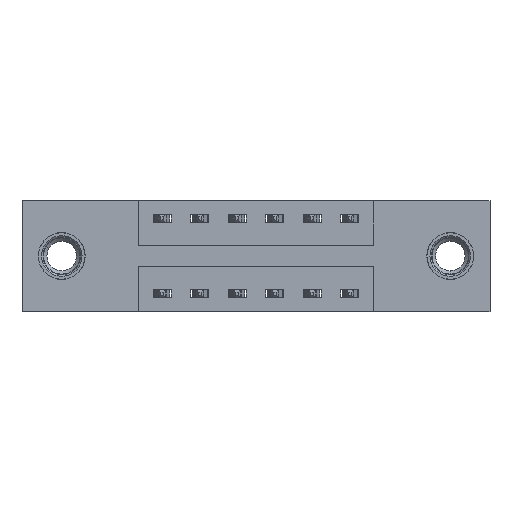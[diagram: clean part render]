
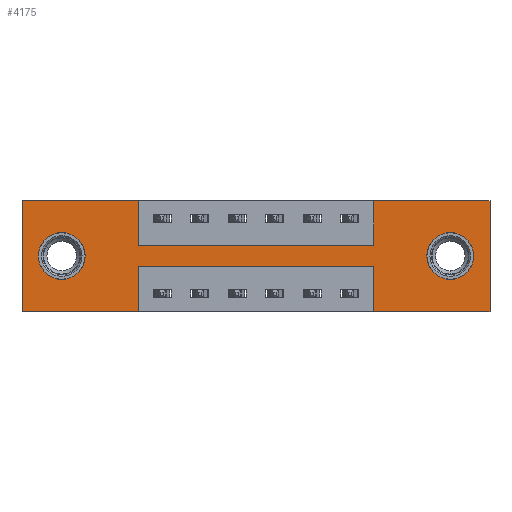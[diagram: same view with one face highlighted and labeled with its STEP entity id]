
A CAD part, front view. The second image highlights one B-rep face of the part: STEP entity #4175.
In plain terms, the highlighted planar face has unit normal (0, -1, 0).
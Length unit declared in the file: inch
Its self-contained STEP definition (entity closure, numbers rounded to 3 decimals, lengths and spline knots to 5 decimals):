
#49 = VERTEX_POINT ( 'NONE', #9052 ) ;
#53 = CARTESIAN_POINT ( 'NONE',  ( 1.1725, 0., -0.37 ) ) ;
#70 = ORIENTED_EDGE ( 'NONE', *, *, #6997, .F. ) ;
#103 = CARTESIAN_POINT ( 'NONE',  ( 1.1725, 0., -0.37 ) ) ;
#174 = VECTOR ( 'NONE', #7941, 39.37008 ) ;
#381 = EDGE_LOOP ( 'NONE', ( #1659, #3938 ) ) ;
#423 = CARTESIAN_POINT ( 'NONE',  ( 0.3875, 0., 0. ) ) ;
#436 = LINE ( 'NONE', #103, #174 ) ;
#499 = EDGE_CURVE ( 'NONE', #2330, #3171, #8116, .T. ) ;
#588 = CARTESIAN_POINT ( 'NONE',  ( 0., 0., 0. ) ) ;
#727 = ORIENTED_EDGE ( 'NONE', *, *, #4081, .F. ) ;
#921 = CARTESIAN_POINT ( 'NONE',  ( 0., 0., 0. ) ) ;
#1027 = PLANE ( 'NONE',  #9394 ) ;
#1106 = CARTESIAN_POINT ( 'NONE',  ( 0., 0., 0. ) ) ;
#1141 = EDGE_CURVE ( 'NONE', #3171, #2044, #2951, .T. ) ;
#1189 = AXIS2_PLACEMENT_3D ( 'NONE', #4025, #9330, #4783 ) ;
#1197 = VECTOR ( 'NONE', #1603, 39.37008 ) ;
#1314 = CARTESIAN_POINT ( 'NONE',  ( 0.3875, 0., 0. ) ) ;
#1422 = CARTESIAN_POINT ( 'NONE',  ( 0., 0., -0.37 ) ) ;
#1438 = FACE_BOUND ( 'NONE', #3781, .T. ) ;
#1603 = DIRECTION ( 'NONE',  ( -1., 0., 0. ) ) ;
#1659 = ORIENTED_EDGE ( 'NONE', *, *, #3507, .T. ) ;
#1663 = VERTEX_POINT ( 'NONE', #9031 ) ;
#1682 = FACE_BOUND ( 'NONE', #381, .T. ) ;
#1936 = ORIENTED_EDGE ( 'NONE', *, *, #4404, .T. ) ;
#2023 = EDGE_LOOP ( 'NONE', ( #3216, #3951, #70, #6258, #3240, #6287, #5935, #3322, #2630, #2986, #727, #7755 ) ) ;
#2044 = VERTEX_POINT ( 'NONE', #6696 ) ;
#2163 = DIRECTION ( 'NONE',  ( 0., 1., 0. ) ) ;
#2310 = VECTOR ( 'NONE', #8249, 39.37008 ) ;
#2313 = LINE ( 'NONE', #5577, #5993 ) ;
#2330 = VERTEX_POINT ( 'NONE', #3100 ) ;
#2378 = DIRECTION ( 'NONE',  ( -1., 0., 0. ) ) ;
#2382 = DIRECTION ( 'NONE',  ( 0., 0., 1. ) ) ;
#2519 = VERTEX_POINT ( 'NONE', #3971 ) ;
#2527 = CARTESIAN_POINT ( 'NONE',  ( 0.3875, 0., -0.22 ) ) ;
#2543 = LINE ( 'NONE', #1314, #2310 ) ;
#2621 = DIRECTION ( 'NONE',  ( 0., 0., -1. ) ) ;
#2630 = ORIENTED_EDGE ( 'NONE', *, *, #9850, .F. ) ;
#2774 = CARTESIAN_POINT ( 'NONE',  ( 1.1725, 0., 0. ) ) ;
#2812 = LINE ( 'NONE', #6273, #1197 ) ;
#2837 = VERTEX_POINT ( 'NONE', #423 ) ;
#2890 = CARTESIAN_POINT ( 'NONE',  ( 0.1325, 0., -0.263 ) ) ;
#2951 = LINE ( 'NONE', #1106, #6819 ) ;
#2986 = ORIENTED_EDGE ( 'NONE', *, *, #3073, .F. ) ;
#3073 = EDGE_CURVE ( 'NONE', #9194, #2837, #8649, .T. ) ;
#3100 = CARTESIAN_POINT ( 'NONE',  ( 1.1725, 0., -0.15 ) ) ;
#3124 = DIRECTION ( 'NONE',  ( 1., 0., 0. ) ) ;
#3140 = VERTEX_POINT ( 'NONE', #4718 ) ;
#3171 = VERTEX_POINT ( 'NONE', #4756 ) ;
#3194 = EDGE_CURVE ( 'NONE', #2044, #7937, #2313, .T. ) ;
#3216 = ORIENTED_EDGE ( 'NONE', *, *, #5064, .F. ) ;
#3240 = ORIENTED_EDGE ( 'NONE', *, *, #3194, .F. ) ;
#3246 = VECTOR ( 'NONE', #9794, 39.37008 ) ;
#3322 = ORIENTED_EDGE ( 'NONE', *, *, #6348, .F. ) ;
#3371 = CIRCLE ( 'NONE', #8724, 0.078 ) ;
#3507 = EDGE_CURVE ( 'NONE', #5974, #2519, #8302, .T. ) ;
#3514 = CARTESIAN_POINT ( 'NONE',  ( 1.4275, 0., -0.185 ) ) ;
#3628 = VERTEX_POINT ( 'NONE', #2890 ) ;
#3651 = CARTESIAN_POINT ( 'NONE',  ( 0.1325, 0., -0.185 ) ) ;
#3781 = EDGE_LOOP ( 'NONE', ( #1936, #8910 ) ) ;
#3938 = ORIENTED_EDGE ( 'NONE', *, *, #6304, .T. ) ;
#3951 = ORIENTED_EDGE ( 'NONE', *, *, #8010, .F. ) ;
#3971 = CARTESIAN_POINT ( 'NONE',  ( 1.4275, 0., -0.263 ) ) ;
#4025 = CARTESIAN_POINT ( 'NONE',  ( 1.4275, 0., -0.185 ) ) ;
#4081 = EDGE_CURVE ( 'NONE', #3140, #9194, #6538, .T. ) ;
#4086 = VERTEX_POINT ( 'NONE', #2527 ) ;
#4138 = AXIS2_PLACEMENT_3D ( 'NONE', #3651, #8980, #4425 ) ;
#4175 = ADVANCED_FACE ( 'NONE', ( #1682, #1438, #9541 ), #1027, .T. ) ;
#4288 = DIRECTION ( 'NONE',  ( 0., 0., -1. ) ) ;
#4404 = EDGE_CURVE ( 'NONE', #6648, #3628, #3371, .T. ) ;
#4425 = DIRECTION ( 'NONE',  ( 0., 0., 1. ) ) ;
#4718 = CARTESIAN_POINT ( 'NONE',  ( 0., 0., -0.37 ) ) ;
#4756 = CARTESIAN_POINT ( 'NONE',  ( 1.1725, 0., 0. ) ) ;
#4783 = DIRECTION ( 'NONE',  ( 0., 0., -1. ) ) ;
#5064 = EDGE_CURVE ( 'NONE', #4086, #1663, #9302, .T. ) ;
#5194 = CARTESIAN_POINT ( 'NONE',  ( 1.4275, 0., -0.107 ) ) ;
#5275 = LINE ( 'NONE', #9237, #7306 ) ;
#5287 = VERTEX_POINT ( 'NONE', #8583 ) ;
#5577 = CARTESIAN_POINT ( 'NONE',  ( 1.56, 0., 0. ) ) ;
#5614 = CARTESIAN_POINT ( 'NONE',  ( 0.3875, 0., -0.15 ) ) ;
#5935 = ORIENTED_EDGE ( 'NONE', *, *, #499, .F. ) ;
#5974 = VERTEX_POINT ( 'NONE', #5194 ) ;
#5993 = VECTOR ( 'NONE', #7813, 39.37008 ) ;
#6112 = DIRECTION ( 'NONE',  ( -1., 0., 0. ) ) ;
#6150 = VECTOR ( 'NONE', #2382, 39.37008 ) ;
#6206 = EDGE_CURVE ( 'NONE', #7937, #9544, #5275, .T. ) ;
#6215 = CARTESIAN_POINT ( 'NONE',  ( 1.56, 0., -0.37 ) ) ;
#6258 = ORIENTED_EDGE ( 'NONE', *, *, #6206, .F. ) ;
#6273 = CARTESIAN_POINT ( 'NONE',  ( 0.3875, 0., -0.22 ) ) ;
#6287 = ORIENTED_EDGE ( 'NONE', *, *, #1141, .F. ) ;
#6304 = EDGE_CURVE ( 'NONE', #2519, #5974, #6848, .T. ) ;
#6348 = EDGE_CURVE ( 'NONE', #49, #2330, #8588, .T. ) ;
#6386 = VECTOR ( 'NONE', #7127, 39.37008 ) ;
#6497 = CARTESIAN_POINT ( 'NONE',  ( 0., 0., -0.37 ) ) ;
#6538 = LINE ( 'NONE', #921, #8061 ) ;
#6628 = EDGE_CURVE ( 'NONE', #3628, #6648, #8007, .T. ) ;
#6648 = VERTEX_POINT ( 'NONE', #6773 ) ;
#6672 = VECTOR ( 'NONE', #3124, 39.37008 ) ;
#6696 = CARTESIAN_POINT ( 'NONE',  ( 1.56, 0., 0. ) ) ;
#6773 = CARTESIAN_POINT ( 'NONE',  ( 0.1325, 0., -0.107 ) ) ;
#6797 = CARTESIAN_POINT ( 'NONE',  ( 0.1325, 0., -0.185 ) ) ;
#6819 = VECTOR ( 'NONE', #7026, 39.37008 ) ;
#6848 = CIRCLE ( 'NONE', #1189, 0.078 ) ;
#6997 = EDGE_CURVE ( 'NONE', #9544, #5287, #436, .T. ) ;
#7026 = DIRECTION ( 'NONE',  ( 1., 0., 0. ) ) ;
#7127 = DIRECTION ( 'NONE',  ( 1., 0., 0. ) ) ;
#7148 = DIRECTION ( 'NONE',  ( 0., 0., 1. ) ) ;
#7245 = DIRECTION ( 'NONE',  ( 0., -1., 0. ) ) ;
#7306 = VECTOR ( 'NONE', #2378, 39.37008 ) ;
#7539 = DIRECTION ( 'NONE',  ( 0., 0., 1. ) ) ;
#7717 = VECTOR ( 'NONE', #6112, 39.37008 ) ;
#7755 = ORIENTED_EDGE ( 'NONE', *, *, #9951, .F. ) ;
#7813 = DIRECTION ( 'NONE',  ( 0., 0., -1. ) ) ;
#7937 = VERTEX_POINT ( 'NONE', #6215 ) ;
#7941 = DIRECTION ( 'NONE',  ( 0., 0., 1. ) ) ;
#8007 = CIRCLE ( 'NONE', #4138, 0.078 ) ;
#8010 = EDGE_CURVE ( 'NONE', #5287, #4086, #2812, .T. ) ;
#8061 = VECTOR ( 'NONE', #7148, 39.37008 ) ;
#8116 = LINE ( 'NONE', #2774, #6150 ) ;
#8249 = DIRECTION ( 'NONE',  ( 0., 0., -1. ) ) ;
#8302 = CIRCLE ( 'NONE', #9755, 0.078 ) ;
#8474 = CARTESIAN_POINT ( 'NONE',  ( 0., 0., 0. ) ) ;
#8583 = CARTESIAN_POINT ( 'NONE',  ( 1.1725, 0., -0.22 ) ) ;
#8588 = LINE ( 'NONE', #5614, #6386 ) ;
#8649 = LINE ( 'NONE', #8474, #6672 ) ;
#8724 = AXIS2_PLACEMENT_3D ( 'NONE', #6797, #2163, #7539 ) ;
#8850 = DIRECTION ( 'NONE',  ( 0., 1., 0. ) ) ;
#8910 = ORIENTED_EDGE ( 'NONE', *, *, #6628, .T. ) ;
#8980 = DIRECTION ( 'NONE',  ( 0., 1., 0. ) ) ;
#9031 = CARTESIAN_POINT ( 'NONE',  ( 0.3875, 0., -0.37 ) ) ;
#9052 = CARTESIAN_POINT ( 'NONE',  ( 0.3875, 0., -0.15 ) ) ;
#9077 = CARTESIAN_POINT ( 'NONE',  ( 0.3875, 0., -0.37 ) ) ;
#9194 = VERTEX_POINT ( 'NONE', #588 ) ;
#9237 = CARTESIAN_POINT ( 'NONE',  ( 0., 0., -0.37 ) ) ;
#9302 = LINE ( 'NONE', #9077, #3246 ) ;
#9330 = DIRECTION ( 'NONE',  ( 0., 1., 0. ) ) ;
#9394 = AXIS2_PLACEMENT_3D ( 'NONE', #6497, #7245, #2621 ) ;
#9541 = FACE_OUTER_BOUND ( 'NONE', #2023, .T. ) ;
#9544 = VERTEX_POINT ( 'NONE', #53 ) ;
#9666 = LINE ( 'NONE', #1422, #7717 ) ;
#9755 = AXIS2_PLACEMENT_3D ( 'NONE', #3514, #8850, #4288 ) ;
#9794 = DIRECTION ( 'NONE',  ( 0., 0., -1. ) ) ;
#9850 = EDGE_CURVE ( 'NONE', #2837, #49, #2543, .T. ) ;
#9951 = EDGE_CURVE ( 'NONE', #1663, #3140, #9666, .T. ) ;
